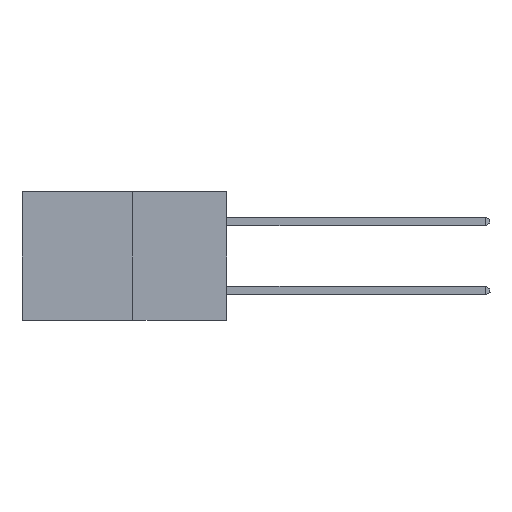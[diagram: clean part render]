
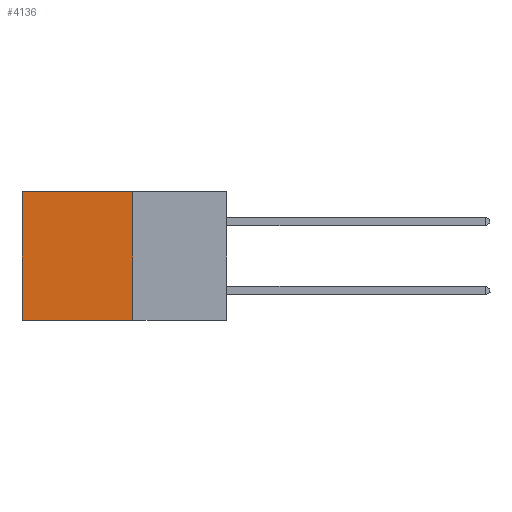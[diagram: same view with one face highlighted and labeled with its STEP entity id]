
A CAD part, left-side view. The second image highlights one B-rep face of the part: STEP entity #4136.
In plain terms, the highlighted planar face has unit normal (-1, 0, 0).
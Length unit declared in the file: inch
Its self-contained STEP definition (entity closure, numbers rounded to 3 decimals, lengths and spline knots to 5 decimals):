
#2224 = DIRECTION ( 'NONE',  ( 0., 1., 0. ) ) ;
#3229 = EDGE_LOOP ( 'NONE', ( #9069, #11113, #21785, #15787 ) ) ;
#4136 = ADVANCED_FACE ( 'NONE', ( #18701 ), #16866, .F. ) ;
#4455 = CARTESIAN_POINT ( 'NONE',  ( 0.277, 0.59, -0.37 ) ) ;
#4591 = DIRECTION ( 'NONE',  ( 0., 0., -1. ) ) ;
#5150 = CARTESIAN_POINT ( 'NONE',  ( 0.277, 0.27, -0.37 ) ) ;
#5326 = VERTEX_POINT ( 'NONE', #5150 ) ;
#5650 = CARTESIAN_POINT ( 'NONE',  ( 0.277, 0.27, -0.37 ) ) ;
#5719 = DIRECTION ( 'NONE',  ( 0., 0., -1. ) ) ;
#5758 = AXIS2_PLACEMENT_3D ( 'NONE', #16498, #13445, #12959 ) ;
#6456 = EDGE_CURVE ( 'NONE', #6986, #5326, #13432, .T. ) ;
#6529 = EDGE_CURVE ( 'NONE', #8917, #16299, #6812, .T. ) ;
#6812 = LINE ( 'NONE', #4455, #22075 ) ;
#6986 = VERTEX_POINT ( 'NONE', #16780 ) ;
#8256 = DIRECTION ( 'NONE',  ( 0., 1., 0. ) ) ;
#8673 = LINE ( 'NONE', #8749, #22776 ) ;
#8749 = CARTESIAN_POINT ( 'NONE',  ( 0.277, 0.27, -0.37 ) ) ;
#8917 = VERTEX_POINT ( 'NONE', #9101 ) ;
#9069 = ORIENTED_EDGE ( 'NONE', *, *, #6529, .T. ) ;
#9101 = CARTESIAN_POINT ( 'NONE',  ( 0.277, 0.59, 0. ) ) ;
#10524 = EDGE_CURVE ( 'NONE', #5326, #16299, #8673, .T. ) ;
#11113 = ORIENTED_EDGE ( 'NONE', *, *, #10524, .F. ) ;
#12959 = DIRECTION ( 'NONE',  ( 0., 0., -1. ) ) ;
#13285 = EDGE_CURVE ( 'NONE', #6986, #8917, #23206, .T. ) ;
#13432 = LINE ( 'NONE', #5650, #14012 ) ;
#13445 = DIRECTION ( 'NONE',  ( 1., 0., 0. ) ) ;
#13461 = VECTOR ( 'NONE', #2224, 39.37008 ) ;
#14012 = VECTOR ( 'NONE', #5719, 39.37008 ) ;
#15787 = ORIENTED_EDGE ( 'NONE', *, *, #13285, .T. ) ;
#16299 = VERTEX_POINT ( 'NONE', #20993 ) ;
#16498 = CARTESIAN_POINT ( 'NONE',  ( 0.277, 0.27, -0.37 ) ) ;
#16780 = CARTESIAN_POINT ( 'NONE',  ( 0.277, 0.27, 0. ) ) ;
#16866 = PLANE ( 'NONE',  #5758 ) ;
#18701 = FACE_OUTER_BOUND ( 'NONE', #3229, .T. ) ;
#18830 = CARTESIAN_POINT ( 'NONE',  ( 0.277, 0.27, 0. ) ) ;
#20993 = CARTESIAN_POINT ( 'NONE',  ( 0.277, 0.59, -0.37 ) ) ;
#21785 = ORIENTED_EDGE ( 'NONE', *, *, #6456, .F. ) ;
#22075 = VECTOR ( 'NONE', #4591, 39.37008 ) ;
#22776 = VECTOR ( 'NONE', #8256, 39.37008 ) ;
#23206 = LINE ( 'NONE', #18830, #13461 ) ;
